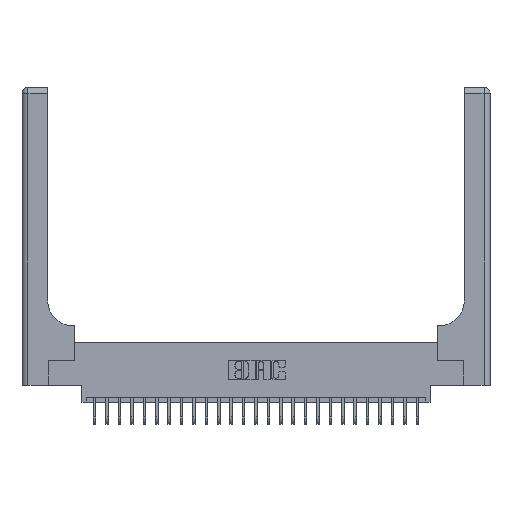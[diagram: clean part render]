
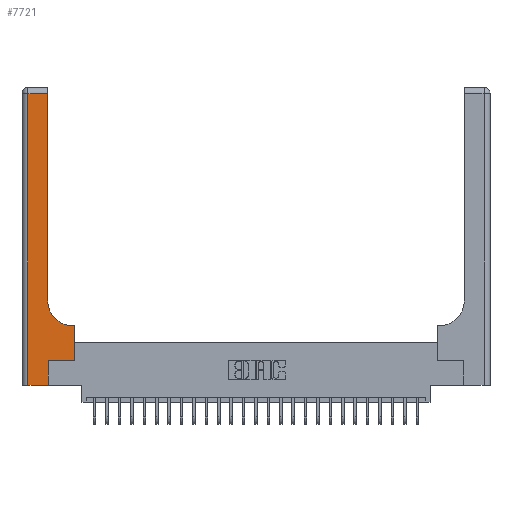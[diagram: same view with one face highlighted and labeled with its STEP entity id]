
A CAD part, top view. The second image highlights one B-rep face of the part: STEP entity #7721.
In plain terms, the highlighted planar face has unit normal (0, 0, 1).
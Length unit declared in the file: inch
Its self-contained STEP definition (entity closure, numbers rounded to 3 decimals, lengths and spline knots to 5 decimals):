
#360 = ORIENTED_EDGE ( 'NONE', *, *, #1379, .T. ) ;
#1159 = DIRECTION ( 'NONE',  ( 0., 0., -1. ) ) ;
#1379 = EDGE_CURVE ( 'NONE', #6618, #26749, #6308, .T. ) ;
#1382 = VECTOR ( 'NONE', #21862, 39.37008 ) ;
#2450 = DIRECTION ( 'NONE',  ( 0., 1., 0. ) ) ;
#2944 = EDGE_CURVE ( 'NONE', #22926, #14163, #3638, .T. ) ;
#3360 = FACE_OUTER_BOUND ( 'NONE', #8152, .T. ) ;
#3638 = LINE ( 'NONE', #11897, #1382 ) ;
#4092 = CARTESIAN_POINT ( 'NONE',  ( 0.528, 0.25, 0.37 ) ) ;
#4171 = DIRECTION ( 'NONE',  ( 0., 1., 0. ) ) ;
#4253 = ORIENTED_EDGE ( 'NONE', *, *, #9709, .T. ) ;
#4491 = VECTOR ( 'NONE', #12174, 39.37008 ) ;
#4601 = VERTEX_POINT ( 'NONE', #23972 ) ;
#4625 = ORIENTED_EDGE ( 'NONE', *, *, #11924, .T. ) ;
#4952 = DIRECTION ( 'NONE',  ( 1., 0., 0. ) ) ;
#4964 = CARTESIAN_POINT ( 'NONE',  ( 0.265, 0., 0.37 ) ) ;
#5390 = CARTESIAN_POINT ( 'NONE',  ( 0., 3., 0.37 ) ) ;
#5431 = CARTESIAN_POINT ( 'NONE',  ( 0.06, 3., 0.37 ) ) ;
#5726 = DIRECTION ( 'NONE',  ( -1., 0., 0. ) ) ;
#6308 = LINE ( 'NONE', #14610, #14007 ) ;
#6618 = VERTEX_POINT ( 'NONE', #4092 ) ;
#6643 = VERTEX_POINT ( 'NONE', #22497 ) ;
#6881 = ORIENTED_EDGE ( 'NONE', *, *, #11818, .T. ) ;
#7404 = VECTOR ( 'NONE', #5726, 39.37008 ) ;
#7542 = PLANE ( 'NONE',  #21579 ) ;
#7721 = ADVANCED_FACE ( 'NONE', ( #3360 ), #7542, .F. ) ;
#8017 = CARTESIAN_POINT ( 'NONE',  ( 0.26, 3., 0.37 ) ) ;
#8152 = EDGE_LOOP ( 'NONE', ( #4253, #19861, #17065, #9050, #4625, #6881, #360, #10225, #10940 ) ) ;
#8846 = EDGE_CURVE ( 'NONE', #26749, #9778, #19085, .T. ) ;
#8996 = CIRCLE ( 'NONE', #11127, 0.25 ) ;
#9050 = ORIENTED_EDGE ( 'NONE', *, *, #2944, .T. ) ;
#9550 = LINE ( 'NONE', #8017, #12144 ) ;
#9709 = EDGE_CURVE ( 'NONE', #22306, #6643, #9550, .T. ) ;
#9778 = VERTEX_POINT ( 'NONE', #22648 ) ;
#9779 = CARTESIAN_POINT ( 'NONE',  ( 0., 2.94, 0.37 ) ) ;
#9864 = CARTESIAN_POINT ( 'NONE',  ( 0.26, 0.6, 0.37 ) ) ;
#10225 = ORIENTED_EDGE ( 'NONE', *, *, #8846, .T. ) ;
#10805 = EDGE_CURVE ( 'NONE', #6643, #23461, #21290, .T. ) ;
#10940 = ORIENTED_EDGE ( 'NONE', *, *, #26614, .T. ) ;
#11127 = AXIS2_PLACEMENT_3D ( 'NONE', #21196, #19350, #4952 ) ;
#11607 = VECTOR ( 'NONE', #13786, 39.37008 ) ;
#11680 = DIRECTION ( 'NONE',  ( -1., 0., 0. ) ) ;
#11818 = EDGE_CURVE ( 'NONE', #4601, #6618, #16053, .T. ) ;
#11897 = CARTESIAN_POINT ( 'NONE',  ( 0., 0., 0.37 ) ) ;
#11924 = EDGE_CURVE ( 'NONE', #14163, #4601, #13513, .T. ) ;
#12144 = VECTOR ( 'NONE', #4171, 39.37008 ) ;
#12174 = DIRECTION ( 'NONE',  ( 1., 0., 0. ) ) ;
#12214 = VECTOR ( 'NONE', #15386, 39.37008 ) ;
#13303 = VECTOR ( 'NONE', #16251, 39.37008 ) ;
#13513 = LINE ( 'NONE', #4964, #12214 ) ;
#13786 = DIRECTION ( 'NONE',  ( 0., -1., 0. ) ) ;
#14007 = VECTOR ( 'NONE', #2450, 39.37008 ) ;
#14163 = VERTEX_POINT ( 'NONE', #16061 ) ;
#14610 = CARTESIAN_POINT ( 'NONE',  ( 0.528, 0.25, 0.37 ) ) ;
#15386 = DIRECTION ( 'NONE',  ( 0., 1., 0. ) ) ;
#15754 = LINE ( 'NONE', #5431, #11607 ) ;
#16053 = LINE ( 'NONE', #16293, #4491 ) ;
#16061 = CARTESIAN_POINT ( 'NONE',  ( 0.265, 0., 0.37 ) ) ;
#16251 = DIRECTION ( 'NONE',  ( -1., 0., 0. ) ) ;
#16293 = CARTESIAN_POINT ( 'NONE',  ( 0.265, 0.25, 0.37 ) ) ;
#17065 = ORIENTED_EDGE ( 'NONE', *, *, #25669, .T. ) ;
#18191 = CARTESIAN_POINT ( 'NONE',  ( 0.26, 0.85, 0.37 ) ) ;
#19085 = LINE ( 'NONE', #9864, #13303 ) ;
#19350 = DIRECTION ( 'NONE',  ( 0., 0., -1. ) ) ;
#19861 = ORIENTED_EDGE ( 'NONE', *, *, #10805, .T. ) ;
#21196 = CARTESIAN_POINT ( 'NONE',  ( 0.51, 0.85, 0.37 ) ) ;
#21290 = LINE ( 'NONE', #9779, #7404 ) ;
#21579 = AXIS2_PLACEMENT_3D ( 'NONE', #5390, #1159, #11680 ) ;
#21862 = DIRECTION ( 'NONE',  ( 1., 0., 0. ) ) ;
#22306 = VERTEX_POINT ( 'NONE', #18191 ) ;
#22497 = CARTESIAN_POINT ( 'NONE',  ( 0.26, 2.94, 0.37 ) ) ;
#22648 = CARTESIAN_POINT ( 'NONE',  ( 0.51, 0.6, 0.37 ) ) ;
#22926 = VERTEX_POINT ( 'NONE', #23632 ) ;
#23461 = VERTEX_POINT ( 'NONE', #23650 ) ;
#23632 = CARTESIAN_POINT ( 'NONE',  ( 0.06, 0., 0.37 ) ) ;
#23650 = CARTESIAN_POINT ( 'NONE',  ( 0.06, 2.94, 0.37 ) ) ;
#23972 = CARTESIAN_POINT ( 'NONE',  ( 0.265, 0.25, 0.37 ) ) ;
#24022 = CARTESIAN_POINT ( 'NONE',  ( 0.528, 0.6, 0.37 ) ) ;
#25669 = EDGE_CURVE ( 'NONE', #23461, #22926, #15754, .T. ) ;
#26614 = EDGE_CURVE ( 'NONE', #9778, #22306, #8996, .T. ) ;
#26749 = VERTEX_POINT ( 'NONE', #24022 ) ;
